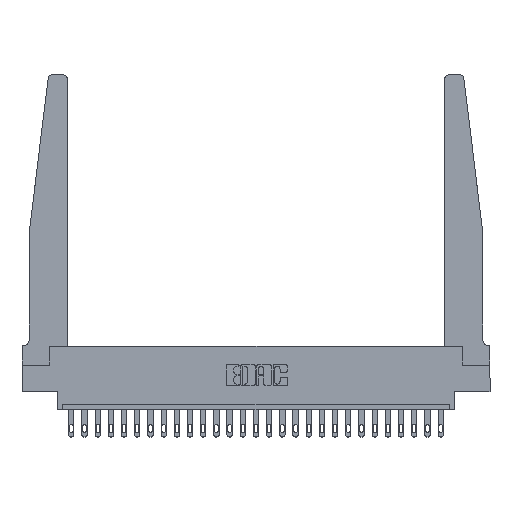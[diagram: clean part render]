
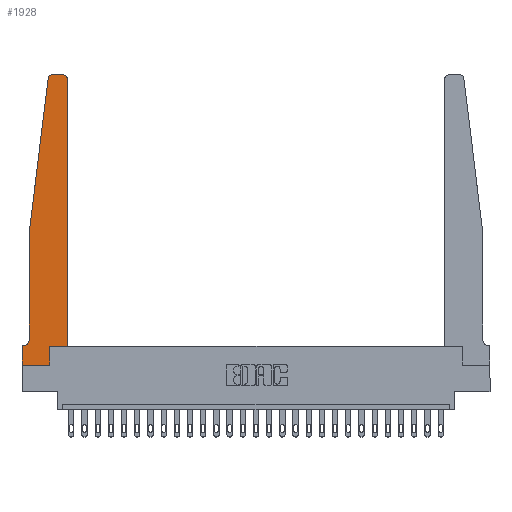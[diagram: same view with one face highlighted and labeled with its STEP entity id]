
A CAD part, top view. The second image highlights one B-rep face of the part: STEP entity #1928.
In plain terms, the highlighted planar face has unit normal (0, 0, 1).
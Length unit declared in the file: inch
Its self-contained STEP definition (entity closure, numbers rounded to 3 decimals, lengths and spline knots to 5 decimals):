
#42 = CARTESIAN_POINT ( 'NONE',  ( 0.425, 0.18, 0.37 ) ) ;
#511 = CARTESIAN_POINT ( 'NONE',  ( 0.065, 1.25, 0.37 ) ) ;
#690 = LINE ( 'NONE', #19812, #11251 ) ;
#938 = VERTEX_POINT ( 'NONE', #13350 ) ;
#1470 = DIRECTION ( 'NONE',  ( 0., 0., 1. ) ) ;
#1639 = AXIS2_PLACEMENT_3D ( 'NONE', #13687, #22941, #2041 ) ;
#1928 = ADVANCED_FACE ( 'NONE', ( #20883 ), #24558, .T. ) ;
#2041 = DIRECTION ( 'NONE',  ( -1., 0., 0. ) ) ;
#2165 = ORIENTED_EDGE ( 'NONE', *, *, #5006, .T. ) ;
#2262 = ORIENTED_EDGE ( 'NONE', *, *, #9019, .T. ) ;
#2271 = LINE ( 'NONE', #4173, #20902 ) ;
#2286 = CARTESIAN_POINT ( 'NONE',  ( 0.015, 0.1875, 0.37 ) ) ;
#2528 = CARTESIAN_POINT ( 'NONE',  ( 0.065, 0.2375, 0.37 ) ) ;
#2772 = ORIENTED_EDGE ( 'NONE', *, *, #21915, .T. ) ;
#3149 = CARTESIAN_POINT ( 'NONE',  ( 0., 0., 0.37 ) ) ;
#3807 = CARTESIAN_POINT ( 'NONE',  ( 0.27653, 2.75, 0.37 ) ) ;
#3947 = LINE ( 'NONE', #7865, #8230 ) ;
#4173 = CARTESIAN_POINT ( 'NONE',  ( 0.425, 0.18, 0.37 ) ) ;
#4252 = EDGE_CURVE ( 'NONE', #16378, #7179, #13926, .T. ) ;
#4260 = LINE ( 'NONE', #21118, #4266 ) ;
#4266 = VECTOR ( 'NONE', #9834, 39.37008 ) ;
#4451 = DIRECTION ( 'NONE',  ( 0., 1., 0. ) ) ;
#4714 = AXIS2_PLACEMENT_3D ( 'NONE', #10882, #18470, #16574 ) ;
#4783 = VERTEX_POINT ( 'NONE', #6408 ) ;
#4937 = DIRECTION ( 'NONE',  ( 0., 0., 1. ) ) ;
#5006 = EDGE_CURVE ( 'NONE', #12255, #7938, #24208, .T. ) ;
#5069 = ORIENTED_EDGE ( 'NONE', *, *, #4252, .T. ) ;
#5193 = ORIENTED_EDGE ( 'NONE', *, *, #13531, .T. ) ;
#5244 = EDGE_LOOP ( 'NONE', ( #18305, #2165, #5193, #15064, #20522, #16782, #2262, #5069, #16689, #2772, #12415, #17686 ) ) ;
#5265 = DIRECTION ( 'NONE',  ( -1., 0., 0. ) ) ;
#5712 = LINE ( 'NONE', #13315, #17982 ) ;
#6102 = CARTESIAN_POINT ( 'NONE',  ( 0.425, 0.18, 0.37 ) ) ;
#6382 = DIRECTION ( 'NONE',  ( 0., 1., 0. ) ) ;
#6408 = CARTESIAN_POINT ( 'NONE',  ( 0.395, 2.75, 0.37 ) ) ;
#7119 = EDGE_CURVE ( 'NONE', #18907, #15037, #9301, .T. ) ;
#7179 = VERTEX_POINT ( 'NONE', #16675 ) ;
#7222 = CARTESIAN_POINT ( 'NONE',  ( 0., 0., 0.37 ) ) ;
#7343 = DIRECTION ( 'NONE',  ( 1., 0., 0. ) ) ;
#7865 = CARTESIAN_POINT ( 'NONE',  ( 0.065, 0.1875, 0.37 ) ) ;
#7938 = VERTEX_POINT ( 'NONE', #23992 ) ;
#8058 = VERTEX_POINT ( 'NONE', #24500 ) ;
#8230 = VECTOR ( 'NONE', #11422, 39.37008 ) ;
#9019 = EDGE_CURVE ( 'NONE', #8058, #16378, #11020, .T. ) ;
#9106 = VECTOR ( 'NONE', #4451, 39.37008 ) ;
#9301 = CIRCLE ( 'NONE', #1639, 0.05 ) ;
#9834 = DIRECTION ( 'NONE',  ( 0., -1., 0. ) ) ;
#9907 = VERTEX_POINT ( 'NONE', #42 ) ;
#10647 = CARTESIAN_POINT ( 'NONE',  ( 0., 0.1875, 0.37 ) ) ;
#10882 = CARTESIAN_POINT ( 'NONE',  ( 0.395, 2.72, 0.37 ) ) ;
#11020 = LINE ( 'NONE', #7222, #11341 ) ;
#11251 = VECTOR ( 'NONE', #6382, 39.37008 ) ;
#11341 = VECTOR ( 'NONE', #14941, 39.37008 ) ;
#11422 = DIRECTION ( 'NONE',  ( -1., 0., 0. ) ) ;
#12255 = VERTEX_POINT ( 'NONE', #3807 ) ;
#12415 = ORIENTED_EDGE ( 'NONE', *, *, #20417, .T. ) ;
#13215 = CIRCLE ( 'NONE', #4714, 0.03 ) ;
#13244 = CARTESIAN_POINT ( 'NONE',  ( 0.27653, 2.72, 0.37 ) ) ;
#13290 = AXIS2_PLACEMENT_3D ( 'NONE', #13244, #1470, #14768 ) ;
#13315 = CARTESIAN_POINT ( 'NONE',  ( 0.065, 1.25, 0.37 ) ) ;
#13350 = CARTESIAN_POINT ( 'NONE',  ( 0.2605, 0.18, 0.37 ) ) ;
#13531 = EDGE_CURVE ( 'NONE', #7938, #21975, #5712, .T. ) ;
#13672 = VERTEX_POINT ( 'NONE', #19758 ) ;
#13687 = CARTESIAN_POINT ( 'NONE',  ( 0.015, 0.2375, 0.37 ) ) ;
#13704 = LINE ( 'NONE', #6102, #9106 ) ;
#13926 = LINE ( 'NONE', #19491, #22664 ) ;
#14768 = DIRECTION ( 'NONE',  ( 1., 0., 0. ) ) ;
#14821 = EDGE_CURVE ( 'NONE', #15037, #8058, #3947, .T. ) ;
#14941 = DIRECTION ( 'NONE',  ( 0., -1., 0. ) ) ;
#15037 = VERTEX_POINT ( 'NONE', #2286 ) ;
#15064 = ORIENTED_EDGE ( 'NONE', *, *, #21263, .T. ) ;
#16378 = VERTEX_POINT ( 'NONE', #3149 ) ;
#16412 = LINE ( 'NONE', #22238, #16580 ) ;
#16574 = DIRECTION ( 'NONE',  ( 1., 0., 0. ) ) ;
#16580 = VECTOR ( 'NONE', #5265, 39.37008 ) ;
#16675 = CARTESIAN_POINT ( 'NONE',  ( 0.2605, 0., 0.37 ) ) ;
#16689 = ORIENTED_EDGE ( 'NONE', *, *, #23382, .T. ) ;
#16782 = ORIENTED_EDGE ( 'NONE', *, *, #14821, .T. ) ;
#17686 = ORIENTED_EDGE ( 'NONE', *, *, #17985, .T. ) ;
#17769 = AXIS2_PLACEMENT_3D ( 'NONE', #10647, #4937, #7343 ) ;
#17982 = VECTOR ( 'NONE', #23311, 39.37008 ) ;
#17985 = EDGE_CURVE ( 'NONE', #13672, #4783, #13215, .T. ) ;
#18305 = ORIENTED_EDGE ( 'NONE', *, *, #24375, .T. ) ;
#18470 = DIRECTION ( 'NONE',  ( 0., 0., 1. ) ) ;
#18907 = VERTEX_POINT ( 'NONE', #2528 ) ;
#19491 = CARTESIAN_POINT ( 'NONE',  ( 0., 0., 0.37 ) ) ;
#19758 = CARTESIAN_POINT ( 'NONE',  ( 0.425, 2.72, 0.37 ) ) ;
#19812 = CARTESIAN_POINT ( 'NONE',  ( 0.2605, 0.18, 0.37 ) ) ;
#20417 = EDGE_CURVE ( 'NONE', #9907, #13672, #13704, .T. ) ;
#20522 = ORIENTED_EDGE ( 'NONE', *, *, #7119, .T. ) ;
#20883 = FACE_OUTER_BOUND ( 'NONE', #5244, .T. ) ;
#20902 = VECTOR ( 'NONE', #23174, 39.37008 ) ;
#21118 = CARTESIAN_POINT ( 'NONE',  ( 0.065, 1.25, 0.37 ) ) ;
#21263 = EDGE_CURVE ( 'NONE', #21975, #18907, #4260, .T. ) ;
#21514 = DIRECTION ( 'NONE',  ( 1., 0., 0. ) ) ;
#21915 = EDGE_CURVE ( 'NONE', #938, #9907, #2271, .T. ) ;
#21975 = VERTEX_POINT ( 'NONE', #511 ) ;
#22238 = CARTESIAN_POINT ( 'NONE',  ( 0.25, 2.75, 0.37 ) ) ;
#22664 = VECTOR ( 'NONE', #21514, 39.37008 ) ;
#22941 = DIRECTION ( 'NONE',  ( 0., 0., -1. ) ) ;
#23174 = DIRECTION ( 'NONE',  ( 1., 0., 0. ) ) ;
#23311 = DIRECTION ( 'NONE',  ( -0.122, -0.992, 0. ) ) ;
#23382 = EDGE_CURVE ( 'NONE', #7179, #938, #690, .T. ) ;
#23992 = CARTESIAN_POINT ( 'NONE',  ( 0.24675, 2.72367, 0.37 ) ) ;
#24208 = CIRCLE ( 'NONE', #13290, 0.03 ) ;
#24375 = EDGE_CURVE ( 'NONE', #4783, #12255, #16412, .T. ) ;
#24500 = CARTESIAN_POINT ( 'NONE',  ( 0., 0.1875, 0.37 ) ) ;
#24558 = PLANE ( 'NONE',  #17769 ) ;
